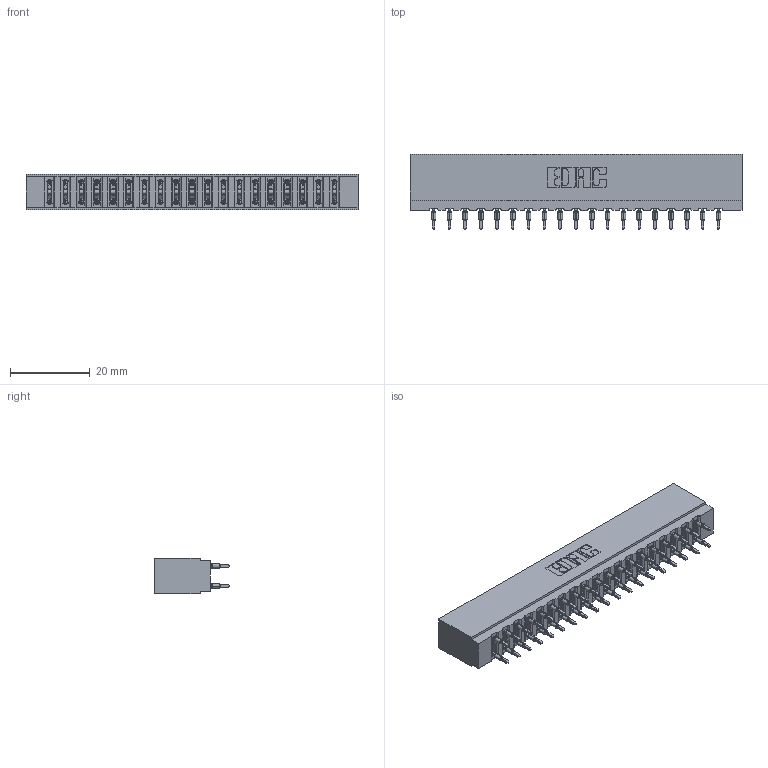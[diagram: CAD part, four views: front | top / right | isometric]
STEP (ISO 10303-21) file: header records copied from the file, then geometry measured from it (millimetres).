
FILE_DESCRIPTION (( 'STEP AP203' ), '1' );
FILE_NAME ('717-038-560-201.STEP', '2026-02-20T17:50:45', ( '' ), ( '' ), 'SwSTEP 2.0', 'SolidWorks 2023', '' );
FILE_SCHEMA (( 'CONFIG_CONTROL_DESIGN' ));
Length unit declared in the file: millimetre
Products named in the file (3): 717-038-560-201; 745-292-001_560; 717 Part_Insulator Option - 06
Assembly tree (39 placements, depth 2):
  717-038-560-201
    717 Part_Insulator Option - 06
    745-292-001_560  x38
Bounding box: 83.16 x 18.78 x 8.89 mm (x, y, z)
Volume: 7441.3 mm3; surface area: 11743 mm2
Topology: 39 solids, 39 shells, 3856 faces, 10549 edges, 6702 vertices
Faces by surface type: plane 2011, cylinder 857, bspline 760, torus 228
Entity records: 36008 total; most frequent: CARTESIAN_POINT 6761, ORIENTED_EDGE 6150, DIRECTION 5395, EDGE_CURVE 3075, VECTOR 2771, LINE 2771, VERTEX_POINT 1966, AXIS2_PLACEMENT_3D 1312
